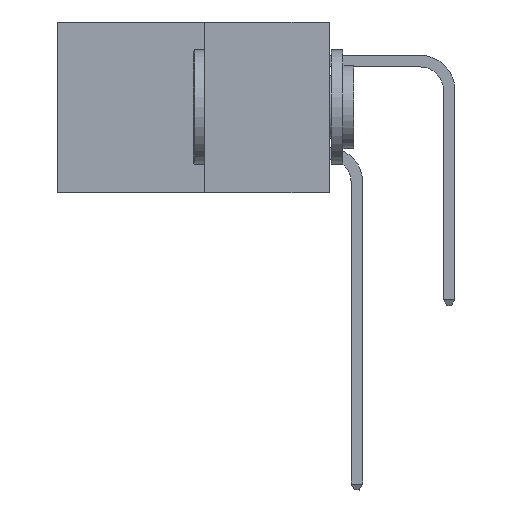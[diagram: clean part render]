
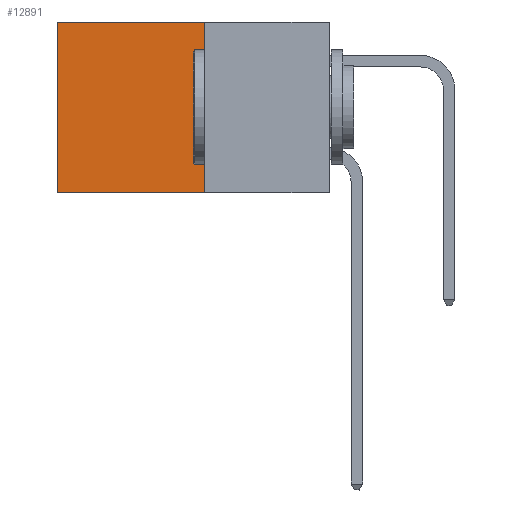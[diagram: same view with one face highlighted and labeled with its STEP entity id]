
A CAD part, left-side view. The second image highlights one B-rep face of the part: STEP entity #12891.
In plain terms, the highlighted planar face has unit normal (-1, 0, 0).
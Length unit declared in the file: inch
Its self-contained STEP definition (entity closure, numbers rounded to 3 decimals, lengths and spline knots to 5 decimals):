
#284 = ORIENTED_EDGE ( 'NONE', *, *, #7865, .T. ) ;
#574 = CARTESIAN_POINT ( 'NONE',  ( 0.277, 0.27, 0. ) ) ;
#886 = EDGE_LOOP ( 'NONE', ( #12860, #5461, #5395, #284 ) ) ;
#1723 = VECTOR ( 'NONE', #18341, 39.37008 ) ;
#3034 = CARTESIAN_POINT ( 'NONE',  ( 0.277, 0.27, -0.37 ) ) ;
#3442 = LINE ( 'NONE', #574, #7728 ) ;
#3900 = EDGE_CURVE ( 'NONE', #13038, #5781, #9675, .T. ) ;
#4326 = CARTESIAN_POINT ( 'NONE',  ( 0.277, 0.59, 0. ) ) ;
#4417 = PLANE ( 'NONE',  #19476 ) ;
#5395 = ORIENTED_EDGE ( 'NONE', *, *, #18847, .F. ) ;
#5457 = VECTOR ( 'NONE', #10715, 39.37008 ) ;
#5461 = ORIENTED_EDGE ( 'NONE', *, *, #3900, .F. ) ;
#5536 = VERTEX_POINT ( 'NONE', #20457 ) ;
#5781 = VERTEX_POINT ( 'NONE', #16303 ) ;
#6055 = DIRECTION ( 'NONE',  ( 1., 0., 0. ) ) ;
#6097 = LINE ( 'NONE', #10445, #1723 ) ;
#7031 = CARTESIAN_POINT ( 'NONE',  ( 0.277, 0.59, -0.37 ) ) ;
#7728 = VECTOR ( 'NONE', #13379, 39.37008 ) ;
#7865 = EDGE_CURVE ( 'NONE', #5536, #8689, #3442, .T. ) ;
#8632 = DIRECTION ( 'NONE',  ( 0., 0., -1. ) ) ;
#8689 = VERTEX_POINT ( 'NONE', #4326 ) ;
#9319 = FACE_OUTER_BOUND ( 'NONE', #886, .T. ) ;
#9675 = LINE ( 'NONE', #20149, #5457 ) ;
#10445 = CARTESIAN_POINT ( 'NONE',  ( 0.277, 0.27, -0.37 ) ) ;
#10699 = EDGE_CURVE ( 'NONE', #8689, #5781, #17069, .T. ) ;
#10715 = DIRECTION ( 'NONE',  ( 0., 1., 0. ) ) ;
#12860 = ORIENTED_EDGE ( 'NONE', *, *, #10699, .T. ) ;
#12891 = ADVANCED_FACE ( 'NONE', ( #9319 ), #4417, .F. ) ;
#13038 = VERTEX_POINT ( 'NONE', #3034 ) ;
#13379 = DIRECTION ( 'NONE',  ( 0., 1., 0. ) ) ;
#15501 = CARTESIAN_POINT ( 'NONE',  ( 0.277, 0.27, -0.37 ) ) ;
#16303 = CARTESIAN_POINT ( 'NONE',  ( 0.277, 0.59, -0.37 ) ) ;
#16556 = VECTOR ( 'NONE', #8632, 39.37008 ) ;
#17069 = LINE ( 'NONE', #7031, #16556 ) ;
#17107 = DIRECTION ( 'NONE',  ( 0., 0., -1. ) ) ;
#18341 = DIRECTION ( 'NONE',  ( 0., 0., -1. ) ) ;
#18847 = EDGE_CURVE ( 'NONE', #5536, #13038, #6097, .T. ) ;
#19476 = AXIS2_PLACEMENT_3D ( 'NONE', #15501, #6055, #17107 ) ;
#20149 = CARTESIAN_POINT ( 'NONE',  ( 0.277, 0.27, -0.37 ) ) ;
#20457 = CARTESIAN_POINT ( 'NONE',  ( 0.277, 0.27, 0. ) ) ;
